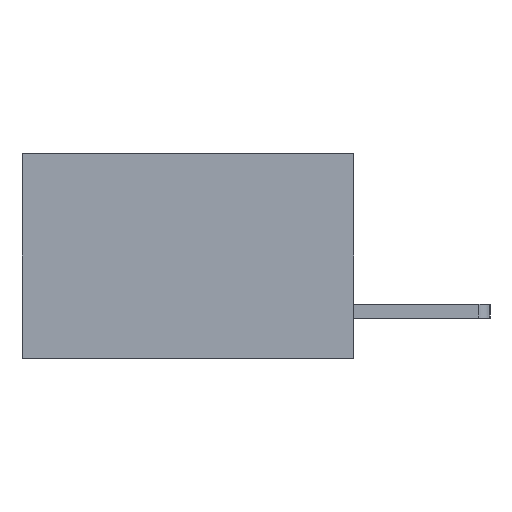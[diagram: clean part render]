
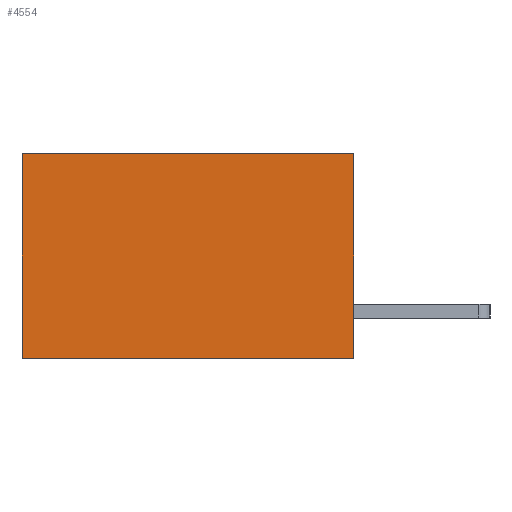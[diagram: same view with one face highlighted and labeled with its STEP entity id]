
A CAD part, left-side view. The second image highlights one B-rep face of the part: STEP entity #4554.
In plain terms, the highlighted planar face has unit normal (-1, 0, 0).
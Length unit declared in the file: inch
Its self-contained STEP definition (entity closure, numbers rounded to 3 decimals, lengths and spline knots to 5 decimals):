
#356 = VERTEX_POINT ( 'NONE', #5822 ) ;
#1228 = EDGE_CURVE ( 'NONE', #2250, #15186, #6934, .T. ) ;
#1471 = DIRECTION ( 'NONE',  ( 0., 0., -1. ) ) ;
#1615 = ORIENTED_EDGE ( 'NONE', *, *, #12266, .F. ) ;
#2017 = VECTOR ( 'NONE', #4617, 39.37008 ) ;
#2250 = VERTEX_POINT ( 'NONE', #3710 ) ;
#2520 = LINE ( 'NONE', #10851, #13422 ) ;
#3710 = CARTESIAN_POINT ( 'NONE',  ( 0.2875, 0., 0. ) ) ;
#3752 = AXIS2_PLACEMENT_3D ( 'NONE', #13030, #14407, #1471 ) ;
#3980 = DIRECTION ( 'NONE',  ( 0., 0., -1. ) ) ;
#4554 = ADVANCED_FACE ( 'NONE', ( #4857 ), #5008, .F. ) ;
#4617 = DIRECTION ( 'NONE',  ( 0., 1., 0. ) ) ;
#4857 = FACE_OUTER_BOUND ( 'NONE', #14183, .T. ) ;
#5008 = PLANE ( 'NONE',  #3752 ) ;
#5822 = CARTESIAN_POINT ( 'NONE',  ( 0.2875, 0., -0.37 ) ) ;
#6225 = CARTESIAN_POINT ( 'NONE',  ( 0.2875, 0.6, 0. ) ) ;
#6853 = EDGE_CURVE ( 'NONE', #15186, #10963, #13980, .T. ) ;
#6934 = LINE ( 'NONE', #12492, #2017 ) ;
#7355 = CARTESIAN_POINT ( 'NONE',  ( 0.2875, 0.6, -0.37 ) ) ;
#8142 = ORIENTED_EDGE ( 'NONE', *, *, #11259, .F. ) ;
#8718 = VECTOR ( 'NONE', #14896, 39.37008 ) ;
#8897 = VECTOR ( 'NONE', #12523, 39.37008 ) ;
#9148 = ORIENTED_EDGE ( 'NONE', *, *, #6853, .T. ) ;
#10202 = LINE ( 'NONE', #12676, #8718 ) ;
#10851 = CARTESIAN_POINT ( 'NONE',  ( 0.2875, 0., 0. ) ) ;
#10963 = VERTEX_POINT ( 'NONE', #7355 ) ;
#11259 = EDGE_CURVE ( 'NONE', #356, #10963, #10202, .T. ) ;
#11292 = CARTESIAN_POINT ( 'NONE',  ( 0.2875, 0.6, 0. ) ) ;
#11320 = ORIENTED_EDGE ( 'NONE', *, *, #1228, .T. ) ;
#12266 = EDGE_CURVE ( 'NONE', #2250, #356, #2520, .T. ) ;
#12492 = CARTESIAN_POINT ( 'NONE',  ( 0.2875, 0., 0. ) ) ;
#12523 = DIRECTION ( 'NONE',  ( 0., 0., -1. ) ) ;
#12676 = CARTESIAN_POINT ( 'NONE',  ( 0.2875, 0., -0.37 ) ) ;
#13030 = CARTESIAN_POINT ( 'NONE',  ( 0.2875, 0., 0. ) ) ;
#13422 = VECTOR ( 'NONE', #3980, 39.37008 ) ;
#13980 = LINE ( 'NONE', #11292, #8897 ) ;
#14183 = EDGE_LOOP ( 'NONE', ( #9148, #8142, #1615, #11320 ) ) ;
#14407 = DIRECTION ( 'NONE',  ( 1., 0., 0. ) ) ;
#14896 = DIRECTION ( 'NONE',  ( 0., 1., 0. ) ) ;
#15186 = VERTEX_POINT ( 'NONE', #6225 ) ;
